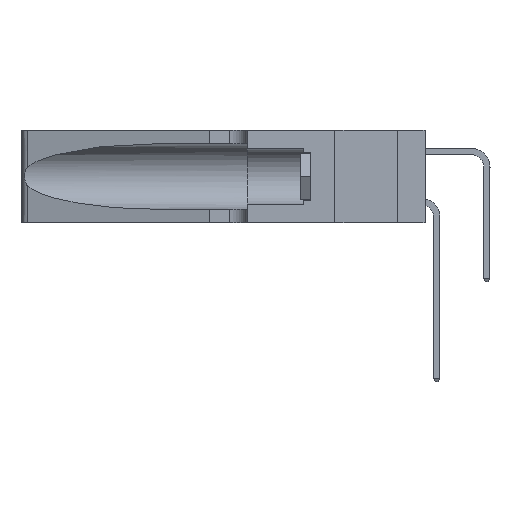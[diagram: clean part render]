
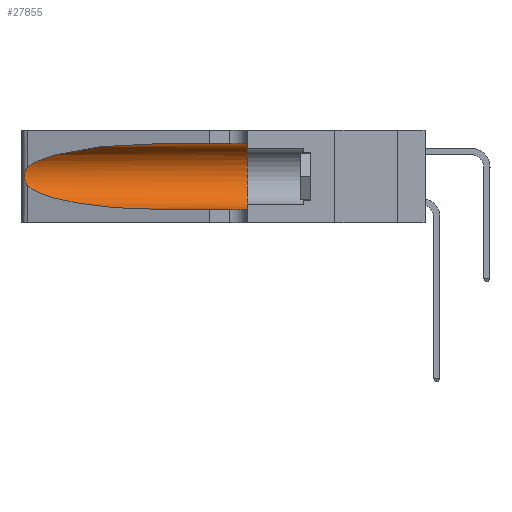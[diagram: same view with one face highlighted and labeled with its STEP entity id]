
A CAD part, left-side view. The second image highlights one B-rep face of the part: STEP entity #27855.
In plain terms, the highlighted cylindrical face has radius 3.308 mm (diameter 6.617 mm), a partial arc.
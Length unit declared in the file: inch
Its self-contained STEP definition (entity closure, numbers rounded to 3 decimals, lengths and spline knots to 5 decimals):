
#234 = LINE ( 'NONE', #1917, #6183 ) ;
#564 = DIRECTION ( 'NONE',  ( 0., 1., 0. ) ) ;
#1917 = CARTESIAN_POINT ( 'NONE',  ( 0.1305, 1.61858, 0.31525 ) ) ;
#2298 = CARTESIAN_POINT ( 'NONE',  ( 0.26075, 1.23896, 0.19203 ) ) ;
#2997 = EDGE_CURVE ( 'NONE', #17243, #14510, #27846, .T. ) ;
#3746 = CYLINDRICAL_SURFACE ( 'NONE', #14634, 0.13025 ) ;
#4476 = EDGE_CURVE ( 'NONE', #18548, #7004, #18922, .T. ) ;
#4719 = CARTESIAN_POINT ( 'NONE',  ( 0.25639, 1.23184, 0.21858 ) ) ;
#4737 = ORIENTED_EDGE ( 'NONE', *, *, #18045, .T. ) ;
#4829 = CARTESIAN_POINT ( 'NONE',  ( 0.26017, 1.23833, 0.17102 ) ) ;
#4837 = CARTESIAN_POINT ( 'NONE',  ( 0.2373, 1.15595, 0.28018 ) ) ;
#5379 = DIRECTION ( 'NONE',  ( 0., -1., 0. ) ) ;
#6124 = EDGE_LOOP ( 'NONE', ( #4737, #25366, #9636, #14368, #13264, #32009 ) ) ;
#6125 = VERTEX_POINT ( 'NONE', #9564 ) ;
#6183 = VECTOR ( 'NONE', #21976, 39.37008 ) ;
#6790 = CARTESIAN_POINT ( 'NONE',  ( 0.25487, 1.22718, 0.22369 ) ) ;
#7004 = VERTEX_POINT ( 'NONE', #20100 ) ;
#7396 = CARTESIAN_POINT ( 'NONE',  ( 0.25789, 1.23486, 0.15765 ) ) ;
#8099 =( BOUNDED_CURVE ( )  B_SPLINE_CURVE ( 3, ( #32203, #17240, #4837, #22368 ),
 .UNSPECIFIED., .F., .F. ) 
 B_SPLINE_CURVE_WITH_KNOTS ( ( 4, 4 ),
 ( 1.5708, 2.84003 ),
 .UNSPECIFIED. ) 
 CURVE ( )  GEOMETRIC_REPRESENTATION_ITEM ( )  RATIONAL_B_SPLINE_CURVE ( ( 1., 0.87, 0.87, 1. ) ) 
 REPRESENTATION_ITEM ( '' )  );
#9013 = CARTESIAN_POINT ( 'NONE',  ( 0.1305, 0.72297, 0.31525 ) ) ;
#9054 = VECTOR ( 'NONE', #5379, 39.37008 ) ;
#9564 = CARTESIAN_POINT ( 'NONE',  ( 0.1305, 0.72297, 0.05475 ) ) ;
#9636 = ORIENTED_EDGE ( 'NONE', *, *, #28384, .T. ) ;
#9922 = CARTESIAN_POINT ( 'NONE',  ( 0.25555, 1.22993, 0.14849 ) ) ;
#10179 = AXIS2_PLACEMENT_3D ( 'NONE', #15623, #564, #18147 ) ;
#10400 = EDGE_CURVE ( 'NONE', #17176, #18548, #234, .T. ) ;
#10558 = CARTESIAN_POINT ( 'NONE',  ( 0.1305, 0.72297, 0.05475 ) ) ;
#11046 = DIRECTION ( 'NONE',  ( 0., -1., 0. ) ) ;
#12857 = CARTESIAN_POINT ( 'NONE',  ( 0.1305, 1.61858, 0.05475 ) ) ;
#13264 = ORIENTED_EDGE ( 'NONE', *, *, #4476, .F. ) ;
#14368 = ORIENTED_EDGE ( 'NONE', *, *, #18769, .T. ) ;
#14510 = VERTEX_POINT ( 'NONE', #31104 ) ;
#14634 = AXIS2_PLACEMENT_3D ( 'NONE', #18457, #11046, #28409 ) ;
#14838 = CARTESIAN_POINT ( 'NONE',  ( 0.25787, 1.23484, 0.2124 ) ) ;
#15623 = CARTESIAN_POINT ( 'NONE',  ( 0.1305, 0.35, 0.185 ) ) ;
#15702 = LINE ( 'NONE', #12857, #9054 ) ;
#17176 = VERTEX_POINT ( 'NONE', #9013 ) ;
#17240 = CARTESIAN_POINT ( 'NONE',  ( 0.18966, 0.96281, 0.31525 ) ) ;
#17243 = VERTEX_POINT ( 'NONE', #6790 ) ;
#17344 = CARTESIAN_POINT ( 'NONE',  ( 0.26018, 1.23835, 0.19895 ) ) ;
#17983 = CARTESIAN_POINT ( 'NONE',  ( 0.25487, 1.22718, 0.14631 ) ) ;
#18045 = EDGE_CURVE ( 'NONE', #17176, #17243, #8099, .T. ) ;
#18147 = DIRECTION ( 'NONE',  ( 0., 0., 1. ) ) ;
#18457 = CARTESIAN_POINT ( 'NONE',  ( 0.1305, 1.61858, 0.185 ) ) ;
#18548 = VERTEX_POINT ( 'NONE', #26990 ) ;
#18769 = EDGE_CURVE ( 'NONE', #6125, #7004, #15702, .T. ) ;
#18922 = CIRCLE ( 'NONE', #10179, 0.13025 ) ;
#19846 = CARTESIAN_POINT ( 'NONE',  ( 0.26075, 1.23896, 0.178 ) ) ;
#20100 = CARTESIAN_POINT ( 'NONE',  ( 0.1305, 0.35, 0.05475 ) ) ;
#20700 =( BOUNDED_CURVE ( )  B_SPLINE_CURVE ( 3, ( #17983, #22994, #25459, #10558 ),
 .UNSPECIFIED., .F., .F. ) 
 B_SPLINE_CURVE_WITH_KNOTS ( ( 4, 4 ),
 ( 3.44316, 4.71239 ),
 .UNSPECIFIED. ) 
 CURVE ( )  GEOMETRIC_REPRESENTATION_ITEM ( )  RATIONAL_B_SPLINE_CURVE ( ( 1., 0.87, 0.87, 1. ) ) 
 REPRESENTATION_ITEM ( '' )  );
#21976 = DIRECTION ( 'NONE',  ( 0., -1., 0. ) ) ;
#22356 = CARTESIAN_POINT ( 'NONE',  ( 0.25856, 1.23593, 0.16098 ) ) ;
#22368 = CARTESIAN_POINT ( 'NONE',  ( 0.25487, 1.22718, 0.22369 ) ) ;
#22994 = CARTESIAN_POINT ( 'NONE',  ( 0.2373, 1.15595, 0.08982 ) ) ;
#24718 = CARTESIAN_POINT ( 'NONE',  ( 0.25555, 1.22994, 0.2215 ) ) ;
#24822 = CARTESIAN_POINT ( 'NONE',  ( 0.25639, 1.23186, 0.15144 ) ) ;
#25366 = ORIENTED_EDGE ( 'NONE', *, *, #2997, .T. ) ;
#25459 = CARTESIAN_POINT ( 'NONE',  ( 0.18966, 0.96281, 0.05475 ) ) ;
#26990 = CARTESIAN_POINT ( 'NONE',  ( 0.1305, 0.35, 0.31525 ) ) ;
#27325 = CARTESIAN_POINT ( 'NONE',  ( 0.25487, 1.22718, 0.14631 ) ) ;
#27846 = B_SPLINE_CURVE_WITH_KNOTS ( 'NONE', 3,
 ( #29695, #24718, #4719, #14838, #32192, #17344, #2298, #19846, #4829, #22356, #7396, #24822, #9922, #27325 ),
 .UNSPECIFIED., .F., .F.,
 ( 4, 2, 2, 2, 2, 2, 4 ),
 ( 0., 0.00027, 0.00053, 0.00107, 0.0016, 0.00187, 0.00214 ),
 .UNSPECIFIED. ) ;
#27855 = ADVANCED_FACE ( 'NONE', ( #30290 ), #3746, .F. ) ;
#28384 = EDGE_CURVE ( 'NONE', #14510, #6125, #20700, .T. ) ;
#28409 = DIRECTION ( 'NONE',  ( 0., 0., -1. ) ) ;
#29695 = CARTESIAN_POINT ( 'NONE',  ( 0.25487, 1.22718, 0.22369 ) ) ;
#30290 = FACE_OUTER_BOUND ( 'NONE', #6124, .T. ) ;
#31104 = CARTESIAN_POINT ( 'NONE',  ( 0.25487, 1.22718, 0.14631 ) ) ;
#32009 = ORIENTED_EDGE ( 'NONE', *, *, #10400, .F. ) ;
#32192 = CARTESIAN_POINT ( 'NONE',  ( 0.25854, 1.2359, 0.20912 ) ) ;
#32203 = CARTESIAN_POINT ( 'NONE',  ( 0.1305, 0.72297, 0.31525 ) ) ;
